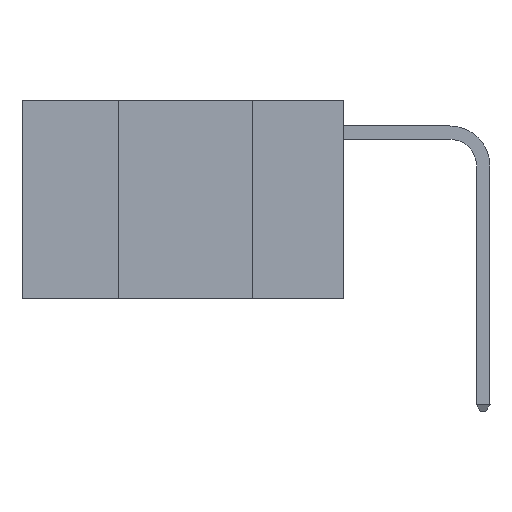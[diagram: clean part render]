
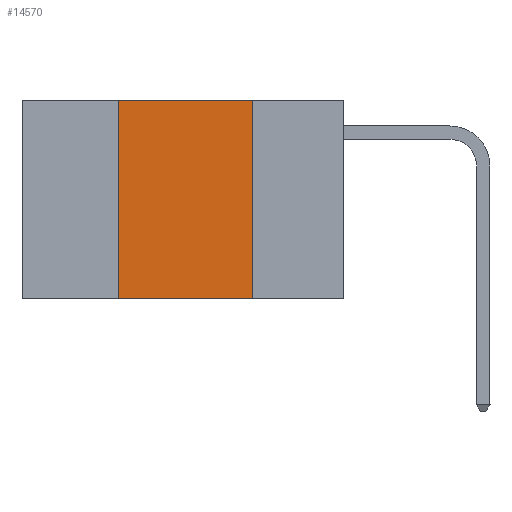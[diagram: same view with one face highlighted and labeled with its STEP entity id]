
A CAD part, left-side view. The second image highlights one B-rep face of the part: STEP entity #14570.
In plain terms, the highlighted planar face has unit normal (-1, 0, 0).
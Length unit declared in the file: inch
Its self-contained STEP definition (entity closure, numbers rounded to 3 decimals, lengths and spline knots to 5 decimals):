
#255 = VECTOR ( 'NONE', #17489, 39.37008 ) ;
#2113 = VERTEX_POINT ( 'NONE', #6870 ) ;
#2731 = CARTESIAN_POINT ( 'NONE',  ( 0., 0.17, -0.37 ) ) ;
#2790 = VERTEX_POINT ( 'NONE', #29351 ) ;
#3244 = EDGE_CURVE ( 'NONE', #23048, #2113, #6424, .T. ) ;
#3937 = ORIENTED_EDGE ( 'NONE', *, *, #27362, .T. ) ;
#5260 = FACE_OUTER_BOUND ( 'NONE', #28781, .T. ) ;
#5369 = CARTESIAN_POINT ( 'NONE',  ( 0., 0.17, 0. ) ) ;
#6386 = VERTEX_POINT ( 'NONE', #2731 ) ;
#6424 = LINE ( 'NONE', #28643, #255 ) ;
#6504 = LINE ( 'NONE', #12948, #23888 ) ;
#6870 = CARTESIAN_POINT ( 'NONE',  ( 0., 0.17, 0. ) ) ;
#7120 = EDGE_CURVE ( 'NONE', #2790, #23048, #25203, .T. ) ;
#7408 = VECTOR ( 'NONE', #19056, 39.37008 ) ;
#8144 = LINE ( 'NONE', #5369, #7408 ) ;
#8654 = EDGE_CURVE ( 'NONE', #2113, #6386, #8144, .T. ) ;
#9870 = DIRECTION ( 'NONE',  ( 0., 0., 1. ) ) ;
#11270 = PLANE ( 'NONE',  #21665 ) ;
#12948 = CARTESIAN_POINT ( 'NONE',  ( 0., 0.6, -0.37 ) ) ;
#14570 = ADVANCED_FACE ( 'NONE', ( #5260 ), #11270, .F. ) ;
#15214 = DIRECTION ( 'NONE',  ( 0., -1., 0. ) ) ;
#15824 = DIRECTION ( 'NONE',  ( 0., 0., -1. ) ) ;
#17489 = DIRECTION ( 'NONE',  ( 0., -1., 0. ) ) ;
#18565 = VECTOR ( 'NONE', #9870, 39.37008 ) ;
#19056 = DIRECTION ( 'NONE',  ( 0., 0., -1. ) ) ;
#19733 = ORIENTED_EDGE ( 'NONE', *, *, #7120, .F. ) ;
#20310 = ORIENTED_EDGE ( 'NONE', *, *, #3244, .F. ) ;
#20801 = CARTESIAN_POINT ( 'NONE',  ( 0., 0.42, 0. ) ) ;
#21665 = AXIS2_PLACEMENT_3D ( 'NONE', #27027, #29273, #15824 ) ;
#23048 = VERTEX_POINT ( 'NONE', #20801 ) ;
#23888 = VECTOR ( 'NONE', #15214, 39.37008 ) ;
#23889 = CARTESIAN_POINT ( 'NONE',  ( 0., 0.42, 0. ) ) ;
#25203 = LINE ( 'NONE', #23889, #18565 ) ;
#25728 = ORIENTED_EDGE ( 'NONE', *, *, #8654, .F. ) ;
#27027 = CARTESIAN_POINT ( 'NONE',  ( 0., 0.6, 0. ) ) ;
#27362 = EDGE_CURVE ( 'NONE', #2790, #6386, #6504, .T. ) ;
#28643 = CARTESIAN_POINT ( 'NONE',  ( 0., 0.6, 0. ) ) ;
#28781 = EDGE_LOOP ( 'NONE', ( #25728, #20310, #19733, #3937 ) ) ;
#29273 = DIRECTION ( 'NONE',  ( 1., 0., 0. ) ) ;
#29351 = CARTESIAN_POINT ( 'NONE',  ( 0., 0.42, -0.37 ) ) ;
